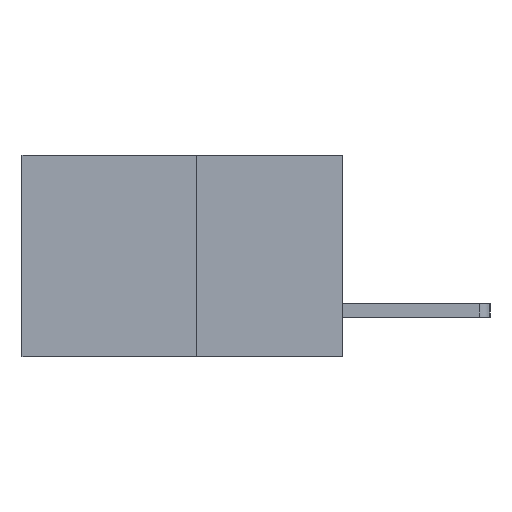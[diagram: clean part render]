
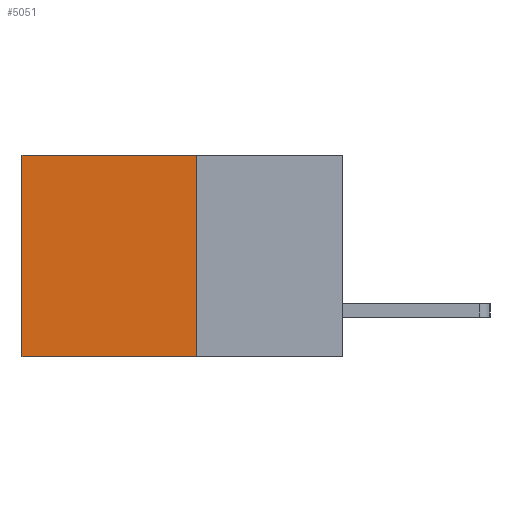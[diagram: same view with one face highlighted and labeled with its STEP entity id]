
A CAD part, left-side view. The second image highlights one B-rep face of the part: STEP entity #5051.
In plain terms, the highlighted planar face has unit normal (-1, 0, 0).
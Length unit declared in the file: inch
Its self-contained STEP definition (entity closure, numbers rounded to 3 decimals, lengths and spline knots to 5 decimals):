
#416 = CARTESIAN_POINT ( 'NONE',  ( 0.277, 0.27, 0. ) ) ;
#615 = ORIENTED_EDGE ( 'NONE', *, *, #9868, .T. ) ;
#1015 = ORIENTED_EDGE ( 'NONE', *, *, #10617, .T. ) ;
#1258 = ORIENTED_EDGE ( 'NONE', *, *, #7539, .F. ) ;
#1287 = ORIENTED_EDGE ( 'NONE', *, *, #10970, .F. ) ;
#1849 = FACE_OUTER_BOUND ( 'NONE', #9445, .T. ) ;
#2842 = CARTESIAN_POINT ( 'NONE',  ( 0.277, 0.27, -0.37 ) ) ;
#2970 = VERTEX_POINT ( 'NONE', #8832 ) ;
#3347 = VECTOR ( 'NONE', #9488, 39.37008 ) ;
#3546 = VERTEX_POINT ( 'NONE', #4915 ) ;
#3718 = LINE ( 'NONE', #2842, #12088 ) ;
#4320 = VECTOR ( 'NONE', #12625, 39.37008 ) ;
#4397 = CARTESIAN_POINT ( 'NONE',  ( 0.277, 0.59, -0.37 ) ) ;
#4915 = CARTESIAN_POINT ( 'NONE',  ( 0.277, 0.27, -0.37 ) ) ;
#5051 = ADVANCED_FACE ( 'NONE', ( #1849 ), #9345, .F. ) ;
#6381 = CARTESIAN_POINT ( 'NONE',  ( 0.277, 0.27, 0. ) ) ;
#6729 = LINE ( 'NONE', #4397, #3347 ) ;
#7539 = EDGE_CURVE ( 'NONE', #3546, #8245, #3718, .T. ) ;
#8245 = VERTEX_POINT ( 'NONE', #12876 ) ;
#8322 = LINE ( 'NONE', #9281, #10683 ) ;
#8832 = CARTESIAN_POINT ( 'NONE',  ( 0.277, 0.59, 0. ) ) ;
#8839 = AXIS2_PLACEMENT_3D ( 'NONE', #9265, #9233, #9218 ) ;
#9218 = DIRECTION ( 'NONE',  ( 0., 0., -1. ) ) ;
#9233 = DIRECTION ( 'NONE',  ( 1., 0., 0. ) ) ;
#9265 = CARTESIAN_POINT ( 'NONE',  ( 0.277, 0.27, -0.37 ) ) ;
#9281 = CARTESIAN_POINT ( 'NONE',  ( 0.277, 0.27, -0.37 ) ) ;
#9345 = PLANE ( 'NONE',  #8839 ) ;
#9445 = EDGE_LOOP ( 'NONE', ( #615, #1258, #1287, #1015 ) ) ;
#9488 = DIRECTION ( 'NONE',  ( 0., 0., -1. ) ) ;
#9868 = EDGE_CURVE ( 'NONE', #2970, #8245, #6729, .T. ) ;
#10012 = DIRECTION ( 'NONE',  ( 0., 1., 0. ) ) ;
#10299 = DIRECTION ( 'NONE',  ( 0., 0., -1. ) ) ;
#10617 = EDGE_CURVE ( 'NONE', #11079, #2970, #12343, .T. ) ;
#10683 = VECTOR ( 'NONE', #10299, 39.37008 ) ;
#10970 = EDGE_CURVE ( 'NONE', #11079, #3546, #8322, .T. ) ;
#11079 = VERTEX_POINT ( 'NONE', #6381 ) ;
#12088 = VECTOR ( 'NONE', #10012, 39.37008 ) ;
#12343 = LINE ( 'NONE', #416, #4320 ) ;
#12625 = DIRECTION ( 'NONE',  ( 0., 1., 0. ) ) ;
#12876 = CARTESIAN_POINT ( 'NONE',  ( 0.277, 0.59, -0.37 ) ) ;
